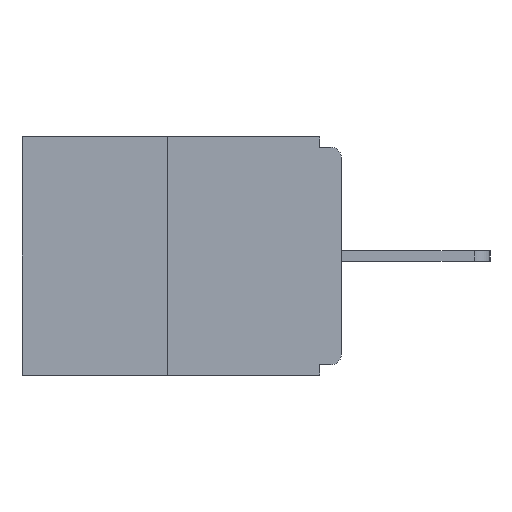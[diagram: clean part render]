
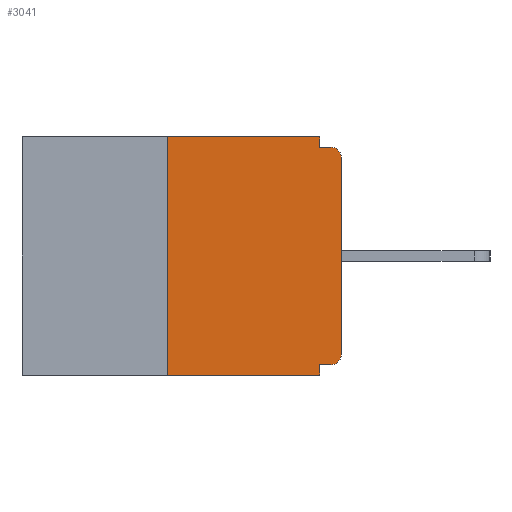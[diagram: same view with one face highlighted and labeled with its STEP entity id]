
A CAD part, left-side view. The second image highlights one B-rep face of the part: STEP entity #3041.
In plain terms, the highlighted planar face has unit normal (-1, 0, 0).
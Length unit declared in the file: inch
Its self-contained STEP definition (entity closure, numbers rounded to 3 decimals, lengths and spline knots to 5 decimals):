
#1069 = LINE ( 'NONE', #13320, #12089 ) ;
#1077 = ORIENTED_EDGE ( 'NONE', *, *, #18809, .F. ) ;
#1122 = DIRECTION ( 'NONE',  ( 0., 0., 1. ) ) ;
#1228 = VECTOR ( 'NONE', #18953, 39.37008 ) ;
#1471 = CARTESIAN_POINT ( 'NONE',  ( 0., 0.031, -0.015 ) ) ;
#1480 = CARTESIAN_POINT ( 'NONE',  ( 0., 0.25, 0. ) ) ;
#1516 = EDGE_CURVE ( 'NONE', #7349, #21030, #15866, .T. ) ;
#1608 = LINE ( 'NONE', #15929, #18407 ) ;
#2462 = VERTEX_POINT ( 'NONE', #16332 ) ;
#3041 = ADVANCED_FACE ( 'NONE', ( #15133 ), #4620, .F. ) ;
#3287 = DIRECTION ( 'NONE',  ( 0., 0., 1. ) ) ;
#3404 = DIRECTION ( 'NONE',  ( 0., -1., 0. ) ) ;
#3514 = EDGE_CURVE ( 'NONE', #20421, #21096, #20246, .T. ) ;
#3516 = CARTESIAN_POINT ( 'NONE',  ( 0., 0.031, -0.343 ) ) ;
#4013 = DIRECTION ( 'NONE',  ( 0., -1., 0. ) ) ;
#4080 = ORIENTED_EDGE ( 'NONE', *, *, #18305, .F. ) ;
#4097 = CARTESIAN_POINT ( 'NONE',  ( 0., 0.25, -0.343 ) ) ;
#4597 = LINE ( 'NONE', #19060, #1228 ) ;
#4620 = PLANE ( 'NONE',  #16151 ) ;
#4711 = CARTESIAN_POINT ( 'NONE',  ( 0., 0.25, 0. ) ) ;
#5361 = LINE ( 'NONE', #19618, #7689 ) ;
#5862 = CARTESIAN_POINT ( 'NONE',  ( 0., 0., -0.328 ) ) ;
#7189 = CARTESIAN_POINT ( 'NONE',  ( 0., 0.015, -0.03 ) ) ;
#7349 = VERTEX_POINT ( 'NONE', #15802 ) ;
#7615 = EDGE_CURVE ( 'NONE', #21096, #19261, #4597, .T. ) ;
#7639 = AXIS2_PLACEMENT_3D ( 'NONE', #15865, #10750, #21614 ) ;
#7689 = VECTOR ( 'NONE', #3404, 39.37008 ) ;
#7828 = CARTESIAN_POINT ( 'NONE',  ( 0., 0.015, -0.015 ) ) ;
#8033 = AXIS2_PLACEMENT_3D ( 'NONE', #7189, #10575, #16054 ) ;
#8940 = VERTEX_POINT ( 'NONE', #1471 ) ;
#9206 = EDGE_CURVE ( 'NONE', #8940, #20586, #19994, .T. ) ;
#9330 = CARTESIAN_POINT ( 'NONE',  ( 0., 0.031, 0. ) ) ;
#9478 = VECTOR ( 'NONE', #4013, 39.37008 ) ;
#9708 = EDGE_CURVE ( 'NONE', #12855, #21513, #1069, .T. ) ;
#10216 = EDGE_CURVE ( 'NONE', #21030, #20586, #17322, .T. ) ;
#10575 = DIRECTION ( 'NONE',  ( -1., 0., 0. ) ) ;
#10693 = DIRECTION ( 'NONE',  ( 0., 0., -1. ) ) ;
#10750 = DIRECTION ( 'NONE',  ( -1., 0., 0. ) ) ;
#11262 = ORIENTED_EDGE ( 'NONE', *, *, #11489, .T. ) ;
#11489 = EDGE_CURVE ( 'NONE', #2462, #7349, #13608, .T. ) ;
#11948 = CARTESIAN_POINT ( 'NONE',  ( 0., 0., -0.03 ) ) ;
#11963 = DIRECTION ( 'NONE',  ( 1., 0., 0. ) ) ;
#12085 = VECTOR ( 'NONE', #21642, 39.37008 ) ;
#12089 = VECTOR ( 'NONE', #19012, 39.37008 ) ;
#12091 = VECTOR ( 'NONE', #3287, 39.37008 ) ;
#12855 = VERTEX_POINT ( 'NONE', #22187 ) ;
#13125 = ORIENTED_EDGE ( 'NONE', *, *, #1516, .T. ) ;
#13218 = CARTESIAN_POINT ( 'NONE',  ( 0., 0., -0.015 ) ) ;
#13320 = CARTESIAN_POINT ( 'NONE',  ( 0., 0.031, -0.343 ) ) ;
#13506 = CARTESIAN_POINT ( 'NONE',  ( 0., 0.46, 0. ) ) ;
#13519 = ORIENTED_EDGE ( 'NONE', *, *, #20322, .T. ) ;
#13608 = CIRCLE ( 'NONE', #7639, 0.015 ) ;
#13727 = DIRECTION ( 'NONE',  ( 0., 0., -1. ) ) ;
#14735 = LINE ( 'NONE', #5862, #12085 ) ;
#15133 = FACE_OUTER_BOUND ( 'NONE', #18446, .T. ) ;
#15802 = CARTESIAN_POINT ( 'NONE',  ( 0., 0., -0.313 ) ) ;
#15865 = CARTESIAN_POINT ( 'NONE',  ( 0., 0.015, -0.313 ) ) ;
#15866 = LINE ( 'NONE', #15989, #12091 ) ;
#15929 = CARTESIAN_POINT ( 'NONE',  ( 0., 0.031, 0. ) ) ;
#15989 = CARTESIAN_POINT ( 'NONE',  ( 0., 0., 0. ) ) ;
#16054 = DIRECTION ( 'NONE',  ( 0., 0., -1. ) ) ;
#16151 = AXIS2_PLACEMENT_3D ( 'NONE', #13506, #11963, #13727 ) ;
#16332 = CARTESIAN_POINT ( 'NONE',  ( 0., 0.015, -0.328 ) ) ;
#17322 = CIRCLE ( 'NONE', #8033, 0.015 ) ;
#18305 = EDGE_CURVE ( 'NONE', #19261, #8940, #1608, .T. ) ;
#18407 = VECTOR ( 'NONE', #10693, 39.37008 ) ;
#18446 = EDGE_LOOP ( 'NONE', ( #21255, #22836, #13519, #18941, #1077, #11262, #13125, #20590, #22310, #4080 ) ) ;
#18809 = EDGE_CURVE ( 'NONE', #2462, #12855, #14735, .T. ) ;
#18941 = ORIENTED_EDGE ( 'NONE', *, *, #9708, .F. ) ;
#18953 = DIRECTION ( 'NONE',  ( 0., -1., 0. ) ) ;
#19012 = DIRECTION ( 'NONE',  ( 0., 0., -1. ) ) ;
#19060 = CARTESIAN_POINT ( 'NONE',  ( 0., 0.46, 0. ) ) ;
#19261 = VERTEX_POINT ( 'NONE', #9330 ) ;
#19618 = CARTESIAN_POINT ( 'NONE',  ( 0., 0.46, -0.343 ) ) ;
#19726 = VECTOR ( 'NONE', #1122, 39.37008 ) ;
#19994 = LINE ( 'NONE', #13218, #9478 ) ;
#20246 = LINE ( 'NONE', #4711, #19726 ) ;
#20322 = EDGE_CURVE ( 'NONE', #20421, #21513, #5361, .T. ) ;
#20421 = VERTEX_POINT ( 'NONE', #4097 ) ;
#20586 = VERTEX_POINT ( 'NONE', #7828 ) ;
#20590 = ORIENTED_EDGE ( 'NONE', *, *, #10216, .T. ) ;
#21030 = VERTEX_POINT ( 'NONE', #11948 ) ;
#21096 = VERTEX_POINT ( 'NONE', #1480 ) ;
#21255 = ORIENTED_EDGE ( 'NONE', *, *, #7615, .F. ) ;
#21513 = VERTEX_POINT ( 'NONE', #3516 ) ;
#21614 = DIRECTION ( 'NONE',  ( 0., 0., -1. ) ) ;
#21642 = DIRECTION ( 'NONE',  ( 0., 1., 0. ) ) ;
#22187 = CARTESIAN_POINT ( 'NONE',  ( 0., 0.031, -0.328 ) ) ;
#22310 = ORIENTED_EDGE ( 'NONE', *, *, #9206, .F. ) ;
#22836 = ORIENTED_EDGE ( 'NONE', *, *, #3514, .F. ) ;
